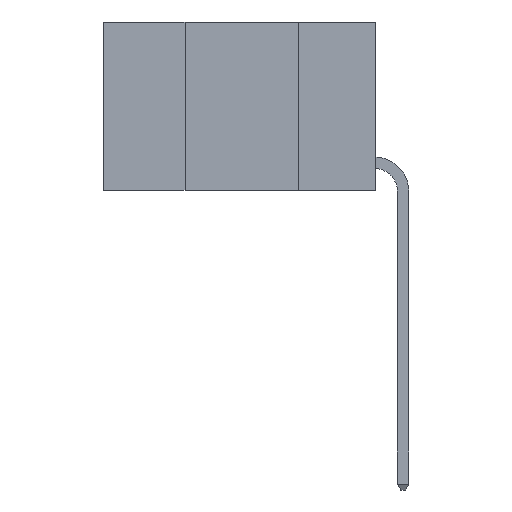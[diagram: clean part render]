
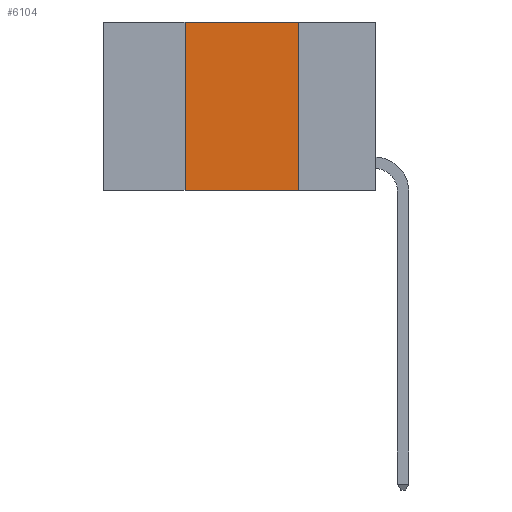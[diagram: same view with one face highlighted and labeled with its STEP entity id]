
A CAD part, left-side view. The second image highlights one B-rep face of the part: STEP entity #6104.
In plain terms, the highlighted planar face has unit normal (-1, 0, 0).
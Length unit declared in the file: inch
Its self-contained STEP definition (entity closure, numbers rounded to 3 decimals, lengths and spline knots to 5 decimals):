
#625 = EDGE_CURVE ( 'NONE', #3473, #7755, #4230, .T. ) ;
#763 = CARTESIAN_POINT ( 'NONE',  ( 0., 0.6, 0. ) ) ;
#1018 = DIRECTION ( 'NONE',  ( 0., -1., 0. ) ) ;
#1059 = CARTESIAN_POINT ( 'NONE',  ( 0., 0.42, 0. ) ) ;
#1163 = EDGE_CURVE ( 'NONE', #3473, #3013, #7017, .T. ) ;
#1451 = FACE_OUTER_BOUND ( 'NONE', #3125, .T. ) ;
#1682 = EDGE_CURVE ( 'NONE', #2667, #7755, #2219, .T. ) ;
#2154 = VECTOR ( 'NONE', #8147, 39.37008 ) ;
#2219 = LINE ( 'NONE', #8301, #2154 ) ;
#2394 = VECTOR ( 'NONE', #1018, 39.37008 ) ;
#2507 = DIRECTION ( 'NONE',  ( 0., -1., 0. ) ) ;
#2667 = VERTEX_POINT ( 'NONE', #2692 ) ;
#2692 = CARTESIAN_POINT ( 'NONE',  ( 0., 0.17, 0. ) ) ;
#2812 = ORIENTED_EDGE ( 'NONE', *, *, #1163, .F. ) ;
#3013 = VERTEX_POINT ( 'NONE', #7598 ) ;
#3125 = EDGE_LOOP ( 'NONE', ( #9125, #7773, #2812, #8914 ) ) ;
#3279 = AXIS2_PLACEMENT_3D ( 'NONE', #763, #8695, #4587 ) ;
#3473 = VERTEX_POINT ( 'NONE', #5203 ) ;
#3804 = VECTOR ( 'NONE', #2507, 39.37008 ) ;
#3840 = PLANE ( 'NONE',  #3279 ) ;
#4230 = LINE ( 'NONE', #6059, #3804 ) ;
#4587 = DIRECTION ( 'NONE',  ( 0., 0., -1. ) ) ;
#5203 = CARTESIAN_POINT ( 'NONE',  ( 0., 0.42, -0.37 ) ) ;
#6059 = CARTESIAN_POINT ( 'NONE',  ( 0., 0.6, -0.37 ) ) ;
#6104 = ADVANCED_FACE ( 'NONE', ( #1451 ), #3840, .F. ) ;
#6782 = VECTOR ( 'NONE', #7622, 39.37008 ) ;
#7017 = LINE ( 'NONE', #1059, #6782 ) ;
#7598 = CARTESIAN_POINT ( 'NONE',  ( 0., 0.42, 0. ) ) ;
#7622 = DIRECTION ( 'NONE',  ( 0., 0., 1. ) ) ;
#7755 = VERTEX_POINT ( 'NONE', #7982 ) ;
#7773 = ORIENTED_EDGE ( 'NONE', *, *, #8673, .F. ) ;
#7982 = CARTESIAN_POINT ( 'NONE',  ( 0., 0.17, -0.37 ) ) ;
#8077 = LINE ( 'NONE', #8892, #2394 ) ;
#8147 = DIRECTION ( 'NONE',  ( 0., 0., -1. ) ) ;
#8301 = CARTESIAN_POINT ( 'NONE',  ( 0., 0.17, 0. ) ) ;
#8673 = EDGE_CURVE ( 'NONE', #3013, #2667, #8077, .T. ) ;
#8695 = DIRECTION ( 'NONE',  ( 1., 0., 0. ) ) ;
#8892 = CARTESIAN_POINT ( 'NONE',  ( 0., 0.6, 0. ) ) ;
#8914 = ORIENTED_EDGE ( 'NONE', *, *, #625, .T. ) ;
#9125 = ORIENTED_EDGE ( 'NONE', *, *, #1682, .F. ) ;
